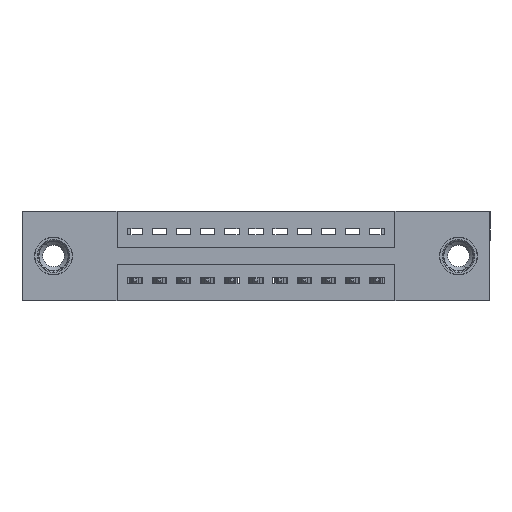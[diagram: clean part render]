
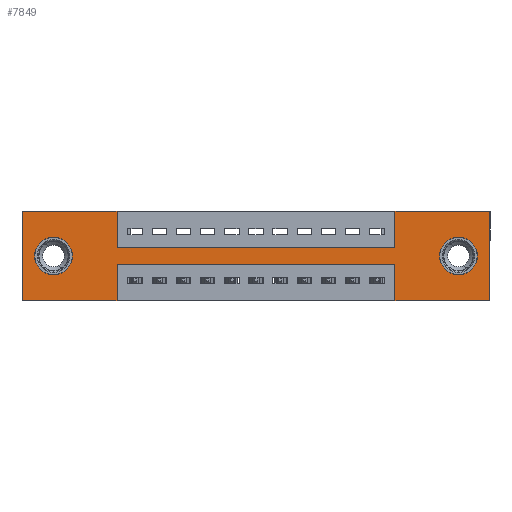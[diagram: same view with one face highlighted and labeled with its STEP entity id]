
A CAD part, front view. The second image highlights one B-rep face of the part: STEP entity #7849.
In plain terms, the highlighted planar face has unit normal (0, -1, 0).
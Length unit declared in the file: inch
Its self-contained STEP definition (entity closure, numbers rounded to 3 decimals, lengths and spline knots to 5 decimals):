
#12 = VERTEX_POINT ( 'NONE', #9481 ) ;
#38 = FACE_OUTER_BOUND ( 'NONE', #2782, .T. ) ;
#298 = DIRECTION ( 'NONE',  ( 0., -1., 0. ) ) ;
#413 = VERTEX_POINT ( 'NONE', #2146 ) ;
#439 = AXIS2_PLACEMENT_3D ( 'NONE', #8195, #298, #2952 ) ;
#628 = VERTEX_POINT ( 'NONE', #9315 ) ;
#1129 = CIRCLE ( 'NONE', #8373, 0.078 ) ;
#1130 = DIRECTION ( 'NONE',  ( 1., 0., 0. ) ) ;
#1445 = ORIENTED_EDGE ( 'NONE', *, *, #5753, .F. ) ;
#1588 = VERTEX_POINT ( 'NONE', #1734 ) ;
#1690 = EDGE_CURVE ( 'NONE', #6483, #413, #10065, .T. ) ;
#1734 = CARTESIAN_POINT ( 'NONE',  ( 1.935, 0., -0.37 ) ) ;
#1969 = VERTEX_POINT ( 'NONE', #6636 ) ;
#1981 = CARTESIAN_POINT ( 'NONE',  ( 0.13, 0., -0.185 ) ) ;
#2146 = CARTESIAN_POINT ( 'NONE',  ( 0.3925, 0., -0.37 ) ) ;
#2168 = ORIENTED_EDGE ( 'NONE', *, *, #12903, .F. ) ;
#2674 = LINE ( 'NONE', #11384, #11777 ) ;
#2782 = EDGE_LOOP ( 'NONE', ( #4754, #6540, #9401, #11067, #15777, #2168, #12694, #5633, #10476, #8404, #1445, #12137 ) ) ;
#2952 = DIRECTION ( 'NONE',  ( 0., 0., -1. ) ) ;
#3019 = EDGE_CURVE ( 'NONE', #8752, #15269, #12279, .T. ) ;
#3189 = CARTESIAN_POINT ( 'NONE',  ( 1.5425, 0., 0. ) ) ;
#3219 = VERTEX_POINT ( 'NONE', #4133 ) ;
#3354 = CARTESIAN_POINT ( 'NONE',  ( 1.5425, 0., -0.15 ) ) ;
#3377 = FACE_BOUND ( 'NONE', #13321, .T. ) ;
#3493 = LINE ( 'NONE', #10287, #10108 ) ;
#3498 = VECTOR ( 'NONE', #15490, 39.37008 ) ;
#3770 = EDGE_LOOP ( 'NONE', ( #9610, #4480 ) ) ;
#3927 = AXIS2_PLACEMENT_3D ( 'NONE', #13443, #12510, #8098 ) ;
#3944 = CARTESIAN_POINT ( 'NONE',  ( 0.3925, 0., -0.22 ) ) ;
#3958 = CIRCLE ( 'NONE', #3927, 0.078 ) ;
#4048 = EDGE_CURVE ( 'NONE', #628, #16488, #14774, .T. ) ;
#4091 = DIRECTION ( 'NONE',  ( 0., 0., -1. ) ) ;
#4133 = CARTESIAN_POINT ( 'NONE',  ( 1.5425, 0., -0.22 ) ) ;
#4310 = CARTESIAN_POINT ( 'NONE',  ( 1.935, 0., 0. ) ) ;
#4480 = ORIENTED_EDGE ( 'NONE', *, *, #13769, .T. ) ;
#4587 = VERTEX_POINT ( 'NONE', #16900 ) ;
#4655 = DIRECTION ( 'NONE',  ( -1., 0., 0. ) ) ;
#4754 = ORIENTED_EDGE ( 'NONE', *, *, #1690, .F. ) ;
#4769 = LINE ( 'NONE', #10557, #9975 ) ;
#4920 = CARTESIAN_POINT ( 'NONE',  ( 0.3925, 0., -0.15 ) ) ;
#5424 = VECTOR ( 'NONE', #1130, 39.37008 ) ;
#5622 = VERTEX_POINT ( 'NONE', #13501 ) ;
#5633 = ORIENTED_EDGE ( 'NONE', *, *, #3019, .F. ) ;
#5722 = EDGE_CURVE ( 'NONE', #16488, #628, #1129, .T. ) ;
#5745 = CARTESIAN_POINT ( 'NONE',  ( 0., 0., 0. ) ) ;
#5753 = EDGE_CURVE ( 'NONE', #11250, #5622, #9825, .T. ) ;
#6153 = CARTESIAN_POINT ( 'NONE',  ( 1.5425, 0., -0.37 ) ) ;
#6345 = LINE ( 'NONE', #6153, #3498 ) ;
#6483 = VERTEX_POINT ( 'NONE', #3944 ) ;
#6540 = ORIENTED_EDGE ( 'NONE', *, *, #15210, .F. ) ;
#6547 = CARTESIAN_POINT ( 'NONE',  ( 0., 0., -0.37 ) ) ;
#6610 = CARTESIAN_POINT ( 'NONE',  ( 0.13, 0., -0.185 ) ) ;
#6636 = CARTESIAN_POINT ( 'NONE',  ( 1.935, 0., 0. ) ) ;
#6970 = CIRCLE ( 'NONE', #15021, 0.078 ) ;
#7106 = DIRECTION ( 'NONE',  ( 0., 1., 0. ) ) ;
#7839 = VECTOR ( 'NONE', #9815, 39.37008 ) ;
#7849 = ADVANCED_FACE ( 'NONE', ( #16031, #3377, #38 ), #16203, .T. ) ;
#8016 = DIRECTION ( 'NONE',  ( -1., 0., 0. ) ) ;
#8098 = DIRECTION ( 'NONE',  ( 0., 0., -1. ) ) ;
#8104 = VECTOR ( 'NONE', #14827, 39.37008 ) ;
#8195 = CARTESIAN_POINT ( 'NONE',  ( 0., 0., -0.37 ) ) ;
#8266 = EDGE_CURVE ( 'NONE', #14166, #8752, #4769, .T. ) ;
#8368 = CARTESIAN_POINT ( 'NONE',  ( 0.3925, 0., -0.37 ) ) ;
#8370 = EDGE_CURVE ( 'NONE', #15269, #15903, #15612, .T. ) ;
#8373 = AXIS2_PLACEMENT_3D ( 'NONE', #1981, #7106, #9962 ) ;
#8404 = ORIENTED_EDGE ( 'NONE', *, *, #15624, .F. ) ;
#8487 = ORIENTED_EDGE ( 'NONE', *, *, #5722, .T. ) ;
#8546 = VERTEX_POINT ( 'NONE', #11182 ) ;
#8752 = VERTEX_POINT ( 'NONE', #4920 ) ;
#8833 = CARTESIAN_POINT ( 'NONE',  ( 0.13, 0., -0.107 ) ) ;
#9192 = DIRECTION ( 'NONE',  ( 0., 0., -1. ) ) ;
#9299 = CARTESIAN_POINT ( 'NONE',  ( 0., 0., -0.37 ) ) ;
#9315 = CARTESIAN_POINT ( 'NONE',  ( 0.13, 0., -0.263 ) ) ;
#9401 = ORIENTED_EDGE ( 'NONE', *, *, #10236, .F. ) ;
#9481 = CARTESIAN_POINT ( 'NONE',  ( 1.805, 0., -0.107 ) ) ;
#9503 = DIRECTION ( 'NONE',  ( 1., 0., 0. ) ) ;
#9610 = ORIENTED_EDGE ( 'NONE', *, *, #10307, .T. ) ;
#9815 = DIRECTION ( 'NONE',  ( -1., 0., 0. ) ) ;
#9825 = LINE ( 'NONE', #5745, #16737 ) ;
#9922 = VECTOR ( 'NONE', #8016, 39.37008 ) ;
#9962 = DIRECTION ( 'NONE',  ( 0., 0., 1. ) ) ;
#9975 = VECTOR ( 'NONE', #4091, 39.37008 ) ;
#10065 = LINE ( 'NONE', #8368, #15897 ) ;
#10108 = VECTOR ( 'NONE', #17139, 39.37008 ) ;
#10236 = EDGE_CURVE ( 'NONE', #8546, #3219, #6345, .T. ) ;
#10287 = CARTESIAN_POINT ( 'NONE',  ( 0., 0., 0. ) ) ;
#10307 = EDGE_CURVE ( 'NONE', #12, #4587, #6970, .T. ) ;
#10476 = ORIENTED_EDGE ( 'NONE', *, *, #8266, .F. ) ;
#10557 = CARTESIAN_POINT ( 'NONE',  ( 0.3925, 0., 0. ) ) ;
#10733 = LINE ( 'NONE', #6547, #9922 ) ;
#11067 = ORIENTED_EDGE ( 'NONE', *, *, #14980, .F. ) ;
#11182 = CARTESIAN_POINT ( 'NONE',  ( 1.5425, 0., -0.37 ) ) ;
#11250 = VERTEX_POINT ( 'NONE', #9299 ) ;
#11384 = CARTESIAN_POINT ( 'NONE',  ( 0.3925, 0., -0.22 ) ) ;
#11678 = CARTESIAN_POINT ( 'NONE',  ( 0.3925, 0., -0.15 ) ) ;
#11777 = VECTOR ( 'NONE', #4655, 39.37008 ) ;
#11785 = CARTESIAN_POINT ( 'NONE',  ( 0., 0., 0. ) ) ;
#11952 = VECTOR ( 'NONE', #9192, 39.37008 ) ;
#12137 = ORIENTED_EDGE ( 'NONE', *, *, #14833, .F. ) ;
#12279 = LINE ( 'NONE', #11678, #5424 ) ;
#12510 = DIRECTION ( 'NONE',  ( 0., 1., 0. ) ) ;
#12571 = LINE ( 'NONE', #4310, #11952 ) ;
#12632 = DIRECTION ( 'NONE',  ( 0., 0., 1. ) ) ;
#12694 = ORIENTED_EDGE ( 'NONE', *, *, #8370, .F. ) ;
#12709 = CARTESIAN_POINT ( 'NONE',  ( 0., 0., -0.37 ) ) ;
#12903 = EDGE_CURVE ( 'NONE', #15903, #1969, #15840, .T. ) ;
#13302 = DIRECTION ( 'NONE',  ( 0., 1., 0. ) ) ;
#13321 = EDGE_LOOP ( 'NONE', ( #8487, #17123 ) ) ;
#13443 = CARTESIAN_POINT ( 'NONE',  ( 1.805, 0., -0.185 ) ) ;
#13461 = CARTESIAN_POINT ( 'NONE',  ( 0.3925, 0., 0. ) ) ;
#13501 = CARTESIAN_POINT ( 'NONE',  ( 0., 0., 0. ) ) ;
#13769 = EDGE_CURVE ( 'NONE', #4587, #12, #3958, .T. ) ;
#13872 = LINE ( 'NONE', #12709, #7839 ) ;
#14166 = VERTEX_POINT ( 'NONE', #13461 ) ;
#14774 = CIRCLE ( 'NONE', #16646, 0.078 ) ;
#14827 = DIRECTION ( 'NONE',  ( 0., 0., 1. ) ) ;
#14833 = EDGE_CURVE ( 'NONE', #413, #11250, #10733, .T. ) ;
#14980 = EDGE_CURVE ( 'NONE', #1588, #8546, #13872, .T. ) ;
#15021 = AXIS2_PLACEMENT_3D ( 'NONE', #15542, #16847, #17014 ) ;
#15210 = EDGE_CURVE ( 'NONE', #3219, #6483, #2674, .T. ) ;
#15269 = VERTEX_POINT ( 'NONE', #3354 ) ;
#15490 = DIRECTION ( 'NONE',  ( 0., 0., 1. ) ) ;
#15542 = CARTESIAN_POINT ( 'NONE',  ( 1.805, 0., -0.185 ) ) ;
#15612 = LINE ( 'NONE', #16308, #8104 ) ;
#15624 = EDGE_CURVE ( 'NONE', #5622, #14166, #3493, .T. ) ;
#15777 = ORIENTED_EDGE ( 'NONE', *, *, #16942, .F. ) ;
#15840 = LINE ( 'NONE', #11785, #17108 ) ;
#15897 = VECTOR ( 'NONE', #16881, 39.37008 ) ;
#15903 = VERTEX_POINT ( 'NONE', #3189 ) ;
#16031 = FACE_BOUND ( 'NONE', #3770, .T. ) ;
#16199 = DIRECTION ( 'NONE',  ( 0., 0., 1. ) ) ;
#16203 = PLANE ( 'NONE',  #439 ) ;
#16308 = CARTESIAN_POINT ( 'NONE',  ( 1.5425, 0., 0. ) ) ;
#16488 = VERTEX_POINT ( 'NONE', #8833 ) ;
#16646 = AXIS2_PLACEMENT_3D ( 'NONE', #6610, #13302, #16199 ) ;
#16737 = VECTOR ( 'NONE', #12632, 39.37008 ) ;
#16847 = DIRECTION ( 'NONE',  ( 0., 1., 0. ) ) ;
#16881 = DIRECTION ( 'NONE',  ( 0., 0., -1. ) ) ;
#16900 = CARTESIAN_POINT ( 'NONE',  ( 1.805, 0., -0.263 ) ) ;
#16942 = EDGE_CURVE ( 'NONE', #1969, #1588, #12571, .T. ) ;
#17014 = DIRECTION ( 'NONE',  ( 0., 0., -1. ) ) ;
#17108 = VECTOR ( 'NONE', #9503, 39.37008 ) ;
#17123 = ORIENTED_EDGE ( 'NONE', *, *, #4048, .T. ) ;
#17139 = DIRECTION ( 'NONE',  ( 1., 0., 0. ) ) ;
